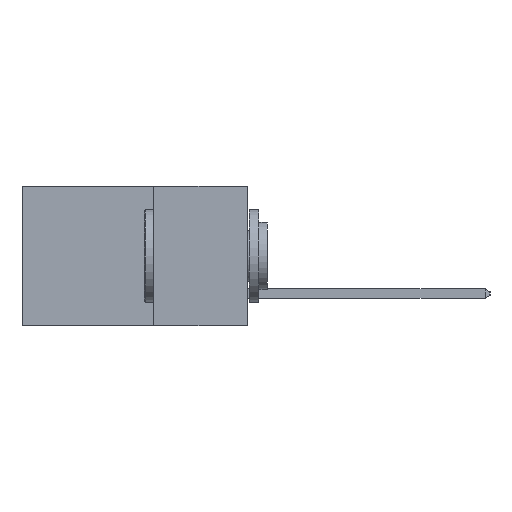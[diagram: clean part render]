
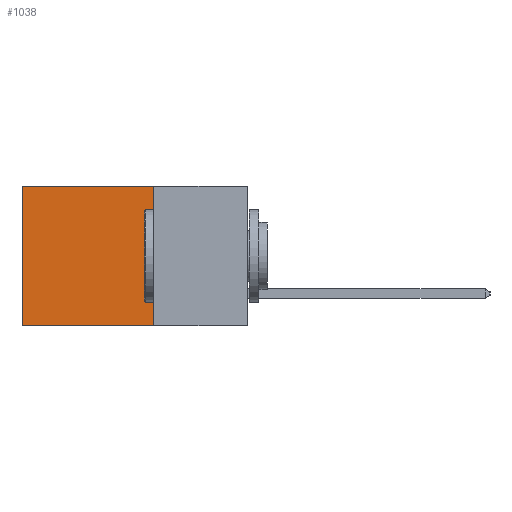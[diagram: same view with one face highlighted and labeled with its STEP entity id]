
A CAD part, left-side view. The second image highlights one B-rep face of the part: STEP entity #1038.
In plain terms, the highlighted planar face has unit normal (-1, 0, 0).
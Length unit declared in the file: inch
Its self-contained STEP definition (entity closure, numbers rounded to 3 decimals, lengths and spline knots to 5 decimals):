
#1038 = ADVANCED_FACE ( 'NONE', ( #3004 ), #4755, .F. ) ;
#1305 = ORIENTED_EDGE ( 'NONE', *, *, #2943, .T. ) ;
#2881 = LINE ( 'NONE', #10316, #10038 ) ;
#2943 = EDGE_CURVE ( 'NONE', #10610, #7900, #17799, .T. ) ;
#3004 = FACE_OUTER_BOUND ( 'NONE', #12921, .T. ) ;
#3248 = VECTOR ( 'NONE', #16443, 39.37008 ) ;
#3632 = ORIENTED_EDGE ( 'NONE', *, *, #4595, .F. ) ;
#3691 = DIRECTION ( 'NONE',  ( 0., 0., -1. ) ) ;
#4197 = AXIS2_PLACEMENT_3D ( 'NONE', #10229, #17958, #3691 ) ;
#4595 = EDGE_CURVE ( 'NONE', #6436, #14646, #2881, .T. ) ;
#4755 = PLANE ( 'NONE',  #4197 ) ;
#6139 = EDGE_CURVE ( 'NONE', #6436, #10610, #9221, .T. ) ;
#6436 = VERTEX_POINT ( 'NONE', #7847 ) ;
#6713 = CARTESIAN_POINT ( 'NONE',  ( 0.2615, 0.25, -0.37 ) ) ;
#7179 = CARTESIAN_POINT ( 'NONE',  ( 0.2615, 0.25, -0.37 ) ) ;
#7688 = CARTESIAN_POINT ( 'NONE',  ( 0.2615, 0.6, 0. ) ) ;
#7847 = CARTESIAN_POINT ( 'NONE',  ( 0.2615, 0.25, 0. ) ) ;
#7900 = VERTEX_POINT ( 'NONE', #17178 ) ;
#9221 = LINE ( 'NONE', #14611, #16771 ) ;
#9858 = VECTOR ( 'NONE', #14378, 39.37008 ) ;
#10038 = VECTOR ( 'NONE', #10291, 39.37008 ) ;
#10229 = CARTESIAN_POINT ( 'NONE',  ( 0.2615, 0.25, -0.37 ) ) ;
#10291 = DIRECTION ( 'NONE',  ( 0., 0., -1. ) ) ;
#10316 = CARTESIAN_POINT ( 'NONE',  ( 0.2615, 0.25, -0.37 ) ) ;
#10610 = VERTEX_POINT ( 'NONE', #7688 ) ;
#11690 = DIRECTION ( 'NONE',  ( 0., 1., 0. ) ) ;
#12329 = LINE ( 'NONE', #7179, #3248 ) ;
#12921 = EDGE_LOOP ( 'NONE', ( #1305, #17460, #3632, #15139 ) ) ;
#14378 = DIRECTION ( 'NONE',  ( 0., 0., -1. ) ) ;
#14461 = CARTESIAN_POINT ( 'NONE',  ( 0.2615, 0.6, -0.37 ) ) ;
#14611 = CARTESIAN_POINT ( 'NONE',  ( 0.2615, 0.25, 0. ) ) ;
#14646 = VERTEX_POINT ( 'NONE', #6713 ) ;
#15139 = ORIENTED_EDGE ( 'NONE', *, *, #6139, .T. ) ;
#16023 = EDGE_CURVE ( 'NONE', #14646, #7900, #12329, .T. ) ;
#16443 = DIRECTION ( 'NONE',  ( 0., 1., 0. ) ) ;
#16771 = VECTOR ( 'NONE', #11690, 39.37008 ) ;
#17178 = CARTESIAN_POINT ( 'NONE',  ( 0.2615, 0.6, -0.37 ) ) ;
#17460 = ORIENTED_EDGE ( 'NONE', *, *, #16023, .F. ) ;
#17799 = LINE ( 'NONE', #14461, #9858 ) ;
#17958 = DIRECTION ( 'NONE',  ( 1., 0., 0. ) ) ;
